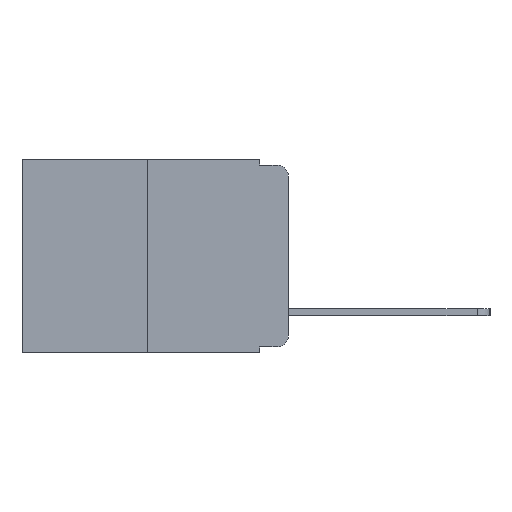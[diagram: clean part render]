
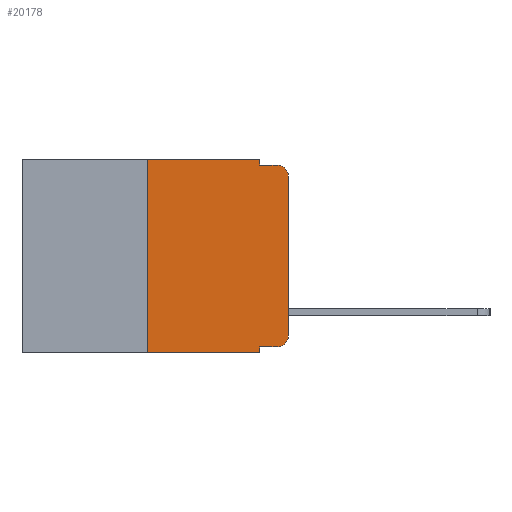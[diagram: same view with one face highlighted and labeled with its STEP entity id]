
A CAD part, left-side view. The second image highlights one B-rep face of the part: STEP entity #20178.
In plain terms, the highlighted planar face has unit normal (-1, 0, 0).
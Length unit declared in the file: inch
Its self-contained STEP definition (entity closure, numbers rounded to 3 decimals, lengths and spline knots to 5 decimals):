
#197 = VECTOR ( 'NONE', #11172, 39.37008 ) ;
#274 = ORIENTED_EDGE ( 'NONE', *, *, #7188, .T. ) ;
#509 = CARTESIAN_POINT ( 'NONE',  ( 0., 0.473, -0.343 ) ) ;
#634 = EDGE_CURVE ( 'NONE', #16814, #3946, #10402, .T. ) ;
#850 = CARTESIAN_POINT ( 'NONE',  ( 0., 0.051, 0. ) ) ;
#968 = CARTESIAN_POINT ( 'NONE',  ( 0., 0.02, -0.313 ) ) ;
#1291 = CARTESIAN_POINT ( 'NONE',  ( 0., 0.473, 0. ) ) ;
#1592 = DIRECTION ( 'NONE',  ( 0., -1., 0. ) ) ;
#1715 = DIRECTION ( 'NONE',  ( 0., 0., -1. ) ) ;
#1827 = ORIENTED_EDGE ( 'NONE', *, *, #13587, .F. ) ;
#1878 = VERTEX_POINT ( 'NONE', #10048 ) ;
#2637 = DIRECTION ( 'NONE',  ( 0., 0., -1. ) ) ;
#2946 = DIRECTION ( 'NONE',  ( 0., 0., -1. ) ) ;
#3003 = EDGE_LOOP ( 'NONE', ( #274, #17039, #5147, #9924, #1827, #10913, #18977, #19450, #3394, #7673 ) ) ;
#3394 = ORIENTED_EDGE ( 'NONE', *, *, #17881, .T. ) ;
#3723 = CARTESIAN_POINT ( 'NONE',  ( 0., 0.051, -0.01 ) ) ;
#3934 = EDGE_CURVE ( 'NONE', #6003, #10318, #13023, .T. ) ;
#3946 = VERTEX_POINT ( 'NONE', #17513 ) ;
#4253 = VECTOR ( 'NONE', #15480, 39.37008 ) ;
#4491 = DIRECTION ( 'NONE',  ( 0., 0., 1. ) ) ;
#4568 = LINE ( 'NONE', #6389, #197 ) ;
#4947 = CARTESIAN_POINT ( 'NONE',  ( 0., 0.473, 0. ) ) ;
#5006 = EDGE_CURVE ( 'NONE', #10318, #7377, #10570, .T. ) ;
#5147 = ORIENTED_EDGE ( 'NONE', *, *, #5006, .F. ) ;
#5808 = VECTOR ( 'NONE', #1592, 39.37008 ) ;
#6003 = VERTEX_POINT ( 'NONE', #19098 ) ;
#6115 = EDGE_CURVE ( 'NONE', #12676, #7377, #7798, .T. ) ;
#6389 = CARTESIAN_POINT ( 'NONE',  ( 0., 0.051, -0.333 ) ) ;
#7188 = EDGE_CURVE ( 'NONE', #14950, #12676, #20208, .T. ) ;
#7377 = VERTEX_POINT ( 'NONE', #12152 ) ;
#7581 = VECTOR ( 'NONE', #14730, 39.37008 ) ;
#7673 = ORIENTED_EDGE ( 'NONE', *, *, #15832, .T. ) ;
#7756 = CARTESIAN_POINT ( 'NONE',  ( 0., 0.051, -0.01 ) ) ;
#7785 = VERTEX_POINT ( 'NONE', #11592 ) ;
#7798 = CIRCLE ( 'NONE', #20042, 0.02 ) ;
#7992 = VECTOR ( 'NONE', #18941, 39.37008 ) ;
#8846 = VECTOR ( 'NONE', #17263, 39.37008 ) ;
#9343 = PLANE ( 'NONE',  #12030 ) ;
#9631 = VECTOR ( 'NONE', #17375, 39.37008 ) ;
#9924 = ORIENTED_EDGE ( 'NONE', *, *, #3934, .F. ) ;
#10048 = CARTESIAN_POINT ( 'NONE',  ( 0., 0.02, -0.333 ) ) ;
#10318 = VERTEX_POINT ( 'NONE', #7756 ) ;
#10402 = LINE ( 'NONE', #10689, #17977 ) ;
#10452 = CARTESIAN_POINT ( 'NONE',  ( 0., 0., -0.313 ) ) ;
#10570 = LINE ( 'NONE', #3723, #5808 ) ;
#10689 = CARTESIAN_POINT ( 'NONE',  ( 0., 0.25, 0. ) ) ;
#10733 = CARTESIAN_POINT ( 'NONE',  ( 0., 0., -0.03 ) ) ;
#10736 = DIRECTION ( 'NONE',  ( -1., 0., 0. ) ) ;
#10913 = ORIENTED_EDGE ( 'NONE', *, *, #634, .F. ) ;
#11172 = DIRECTION ( 'NONE',  ( 0., -1., 0. ) ) ;
#11435 = CARTESIAN_POINT ( 'NONE',  ( 0., 0.25, -0.343 ) ) ;
#11592 = CARTESIAN_POINT ( 'NONE',  ( 0., 0.051, -0.343 ) ) ;
#11886 = CIRCLE ( 'NONE', #19684, 0.02 ) ;
#12030 = AXIS2_PLACEMENT_3D ( 'NONE', #1291, #12512, #2946 ) ;
#12152 = CARTESIAN_POINT ( 'NONE',  ( 0., 0.02, -0.01 ) ) ;
#12212 = DIRECTION ( 'NONE',  ( -1., 0., 0. ) ) ;
#12512 = DIRECTION ( 'NONE',  ( 1., 0., 0. ) ) ;
#12676 = VERTEX_POINT ( 'NONE', #10733 ) ;
#13023 = LINE ( 'NONE', #850, #8846 ) ;
#13188 = LINE ( 'NONE', #19990, #4253 ) ;
#13587 = EDGE_CURVE ( 'NONE', #3946, #6003, #13733, .T. ) ;
#13603 = CARTESIAN_POINT ( 'NONE',  ( 0., 0.02, -0.03 ) ) ;
#13733 = LINE ( 'NONE', #4947, #9631 ) ;
#14730 = DIRECTION ( 'NONE',  ( 0., -1., 0. ) ) ;
#14950 = VERTEX_POINT ( 'NONE', #10452 ) ;
#15480 = DIRECTION ( 'NONE',  ( 0., 0., -1. ) ) ;
#15774 = LINE ( 'NONE', #509, #7581 ) ;
#15832 = EDGE_CURVE ( 'NONE', #1878, #14950, #11886, .T. ) ;
#16140 = FACE_OUTER_BOUND ( 'NONE', #3003, .T. ) ;
#16814 = VERTEX_POINT ( 'NONE', #11435 ) ;
#17039 = ORIENTED_EDGE ( 'NONE', *, *, #6115, .T. ) ;
#17263 = DIRECTION ( 'NONE',  ( 0., 0., -1. ) ) ;
#17375 = DIRECTION ( 'NONE',  ( 0., -1., 0. ) ) ;
#17392 = CARTESIAN_POINT ( 'NONE',  ( 0., 0., 0. ) ) ;
#17513 = CARTESIAN_POINT ( 'NONE',  ( 0., 0.25, 0. ) ) ;
#17605 = CARTESIAN_POINT ( 'NONE',  ( 0., 0.051, -0.333 ) ) ;
#17881 = EDGE_CURVE ( 'NONE', #18681, #1878, #4568, .T. ) ;
#17977 = VECTOR ( 'NONE', #4491, 39.37008 ) ;
#18147 = EDGE_CURVE ( 'NONE', #16814, #7785, #15774, .T. ) ;
#18681 = VERTEX_POINT ( 'NONE', #17605 ) ;
#18916 = EDGE_CURVE ( 'NONE', #18681, #7785, #13188, .T. ) ;
#18941 = DIRECTION ( 'NONE',  ( 0., 0., 1. ) ) ;
#18977 = ORIENTED_EDGE ( 'NONE', *, *, #18147, .T. ) ;
#19098 = CARTESIAN_POINT ( 'NONE',  ( 0., 0.051, 0. ) ) ;
#19450 = ORIENTED_EDGE ( 'NONE', *, *, #18916, .F. ) ;
#19684 = AXIS2_PLACEMENT_3D ( 'NONE', #968, #12212, #2637 ) ;
#19990 = CARTESIAN_POINT ( 'NONE',  ( 0., 0.051, 0. ) ) ;
#20042 = AXIS2_PLACEMENT_3D ( 'NONE', #13603, #10736, #1715 ) ;
#20178 = ADVANCED_FACE ( 'NONE', ( #16140 ), #9343, .F. ) ;
#20208 = LINE ( 'NONE', #17392, #7992 ) ;
